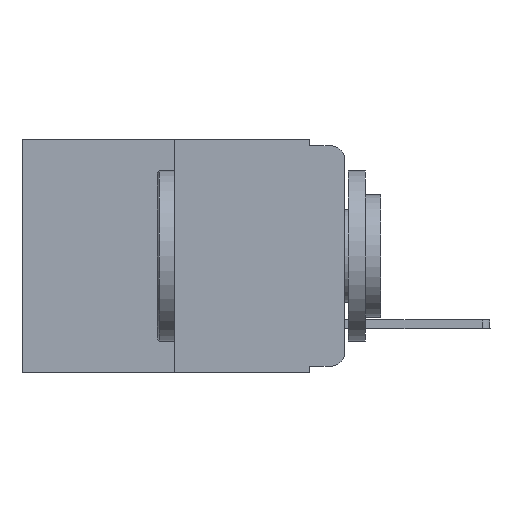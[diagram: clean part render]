
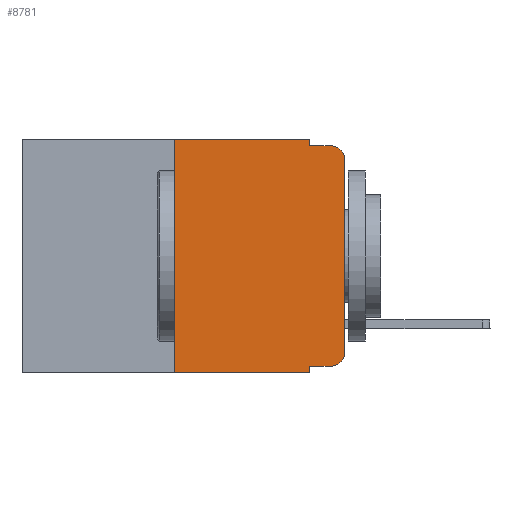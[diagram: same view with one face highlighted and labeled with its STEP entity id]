
A CAD part, left-side view. The second image highlights one B-rep face of the part: STEP entity #8781.
In plain terms, the highlighted planar face has unit normal (-1, 0, 0).
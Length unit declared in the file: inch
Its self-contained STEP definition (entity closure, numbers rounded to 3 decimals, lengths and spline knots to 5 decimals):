
#239 = EDGE_CURVE ( 'NONE', #5263, #3310, #3685, .T. ) ;
#335 = FACE_OUTER_BOUND ( 'NONE', #7612, .T. ) ;
#485 = ORIENTED_EDGE ( 'NONE', *, *, #7658, .T. ) ;
#514 = CARTESIAN_POINT ( 'NONE',  ( 0., 0.051, 0. ) ) ;
#532 = VECTOR ( 'NONE', #7326, 39.37008 ) ;
#600 = ORIENTED_EDGE ( 'NONE', *, *, #5888, .F. ) ;
#647 = AXIS2_PLACEMENT_3D ( 'NONE', #10491, #4248, #7802 ) ;
#681 = CARTESIAN_POINT ( 'NONE',  ( 0., 0.051, -0.333 ) ) ;
#713 = AXIS2_PLACEMENT_3D ( 'NONE', #2343, #8438, #859 ) ;
#859 = DIRECTION ( 'NONE',  ( 0., 0., -1. ) ) ;
#959 = CARTESIAN_POINT ( 'NONE',  ( 0., 0.051, -0.01 ) ) ;
#1010 = CIRCLE ( 'NONE', #3616, 0.02 ) ;
#1040 = VECTOR ( 'NONE', #9550, 39.37008 ) ;
#1182 = CARTESIAN_POINT ( 'NONE',  ( 0., 0.473, 0. ) ) ;
#1304 = CARTESIAN_POINT ( 'NONE',  ( 0., 0., 0. ) ) ;
#1394 = VECTOR ( 'NONE', #2968, 39.37008 ) ;
#1532 = EDGE_CURVE ( 'NONE', #3768, #6406, #4281, .T. ) ;
#1654 = LINE ( 'NONE', #1304, #1394 ) ;
#2176 = VECTOR ( 'NONE', #7659, 39.37008 ) ;
#2260 = CARTESIAN_POINT ( 'NONE',  ( 0., 0.25, -0.343 ) ) ;
#2282 = CARTESIAN_POINT ( 'NONE',  ( 0., 0.051, -0.333 ) ) ;
#2328 = VECTOR ( 'NONE', #6367, 39.37008 ) ;
#2343 = CARTESIAN_POINT ( 'NONE',  ( 0., 0.02, -0.03 ) ) ;
#2379 = DIRECTION ( 'NONE',  ( 0., 0., -1. ) ) ;
#2938 = VERTEX_POINT ( 'NONE', #7392 ) ;
#2962 = CARTESIAN_POINT ( 'NONE',  ( 0., 0.02, -0.333 ) ) ;
#2968 = DIRECTION ( 'NONE',  ( 0., 0., 1. ) ) ;
#2979 = CARTESIAN_POINT ( 'NONE',  ( 0., 0.02, -0.01 ) ) ;
#3271 = EDGE_CURVE ( 'NONE', #6829, #2938, #7675, .T. ) ;
#3310 = VERTEX_POINT ( 'NONE', #5125 ) ;
#3396 = CARTESIAN_POINT ( 'NONE',  ( 0., 0., -0.313 ) ) ;
#3616 = AXIS2_PLACEMENT_3D ( 'NONE', #7581, #11140, #2379 ) ;
#3685 = LINE ( 'NONE', #1182, #532 ) ;
#3768 = VERTEX_POINT ( 'NONE', #7694 ) ;
#3966 = EDGE_CURVE ( 'NONE', #5763, #7145, #1010, .T. ) ;
#4054 = LINE ( 'NONE', #681, #6393 ) ;
#4248 = DIRECTION ( 'NONE',  ( 1., 0., 0. ) ) ;
#4281 = CIRCLE ( 'NONE', #713, 0.02 ) ;
#4326 = EDGE_CURVE ( 'NONE', #6829, #5263, #9485, .T. ) ;
#5077 = VERTEX_POINT ( 'NONE', #959 ) ;
#5125 = CARTESIAN_POINT ( 'NONE',  ( 0., 0.051, 0. ) ) ;
#5263 = VERTEX_POINT ( 'NONE', #9951 ) ;
#5327 = ORIENTED_EDGE ( 'NONE', *, *, #1532, .T. ) ;
#5763 = VERTEX_POINT ( 'NONE', #2962 ) ;
#5888 = EDGE_CURVE ( 'NONE', #3310, #5077, #7680, .T. ) ;
#5932 = DIRECTION ( 'NONE',  ( 0., -1., 0. ) ) ;
#6001 = DIRECTION ( 'NONE',  ( 0., 0., -1. ) ) ;
#6061 = LINE ( 'NONE', #10361, #8684 ) ;
#6113 = ORIENTED_EDGE ( 'NONE', *, *, #11091, .T. ) ;
#6367 = DIRECTION ( 'NONE',  ( 0., 0., 1. ) ) ;
#6393 = VECTOR ( 'NONE', #5932, 39.37008 ) ;
#6406 = VERTEX_POINT ( 'NONE', #2979 ) ;
#6598 = DIRECTION ( 'NONE',  ( 0., -1., 0. ) ) ;
#6829 = VERTEX_POINT ( 'NONE', #2260 ) ;
#6878 = PLANE ( 'NONE',  #647 ) ;
#7057 = ORIENTED_EDGE ( 'NONE', *, *, #3966, .T. ) ;
#7145 = VERTEX_POINT ( 'NONE', #3396 ) ;
#7162 = ORIENTED_EDGE ( 'NONE', *, *, #7758, .F. ) ;
#7326 = DIRECTION ( 'NONE',  ( 0., -1., 0. ) ) ;
#7392 = CARTESIAN_POINT ( 'NONE',  ( 0., 0.051, -0.343 ) ) ;
#7581 = CARTESIAN_POINT ( 'NONE',  ( 0., 0.02, -0.313 ) ) ;
#7612 = EDGE_LOOP ( 'NONE', ( #6113, #5327, #7162, #600, #8149, #9264, #10071, #7941, #485, #7057 ) ) ;
#7658 = EDGE_CURVE ( 'NONE', #9331, #5763, #4054, .T. ) ;
#7659 = DIRECTION ( 'NONE',  ( 0., 0., -1. ) ) ;
#7675 = LINE ( 'NONE', #10099, #10282 ) ;
#7680 = LINE ( 'NONE', #514, #2176 ) ;
#7694 = CARTESIAN_POINT ( 'NONE',  ( 0., 0., -0.03 ) ) ;
#7758 = EDGE_CURVE ( 'NONE', #5077, #6406, #11073, .T. ) ;
#7802 = DIRECTION ( 'NONE',  ( 0., 0., -1. ) ) ;
#7941 = ORIENTED_EDGE ( 'NONE', *, *, #10765, .F. ) ;
#8149 = ORIENTED_EDGE ( 'NONE', *, *, #239, .F. ) ;
#8438 = DIRECTION ( 'NONE',  ( -1., 0., 0. ) ) ;
#8684 = VECTOR ( 'NONE', #6001, 39.37008 ) ;
#8781 = ADVANCED_FACE ( 'NONE', ( #335 ), #6878, .F. ) ;
#9264 = ORIENTED_EDGE ( 'NONE', *, *, #4326, .F. ) ;
#9331 = VERTEX_POINT ( 'NONE', #2282 ) ;
#9485 = LINE ( 'NONE', #10914, #2328 ) ;
#9550 = DIRECTION ( 'NONE',  ( 0., -1., 0. ) ) ;
#9780 = CARTESIAN_POINT ( 'NONE',  ( 0., 0.051, -0.01 ) ) ;
#9951 = CARTESIAN_POINT ( 'NONE',  ( 0., 0.25, 0. ) ) ;
#10071 = ORIENTED_EDGE ( 'NONE', *, *, #3271, .T. ) ;
#10099 = CARTESIAN_POINT ( 'NONE',  ( 0., 0.473, -0.343 ) ) ;
#10282 = VECTOR ( 'NONE', #6598, 39.37008 ) ;
#10361 = CARTESIAN_POINT ( 'NONE',  ( 0., 0.051, 0. ) ) ;
#10491 = CARTESIAN_POINT ( 'NONE',  ( 0., 0.473, 0. ) ) ;
#10765 = EDGE_CURVE ( 'NONE', #9331, #2938, #6061, .T. ) ;
#10914 = CARTESIAN_POINT ( 'NONE',  ( 0., 0.25, 0. ) ) ;
#11073 = LINE ( 'NONE', #9780, #1040 ) ;
#11091 = EDGE_CURVE ( 'NONE', #7145, #3768, #1654, .T. ) ;
#11140 = DIRECTION ( 'NONE',  ( -1., 0., 0. ) ) ;
